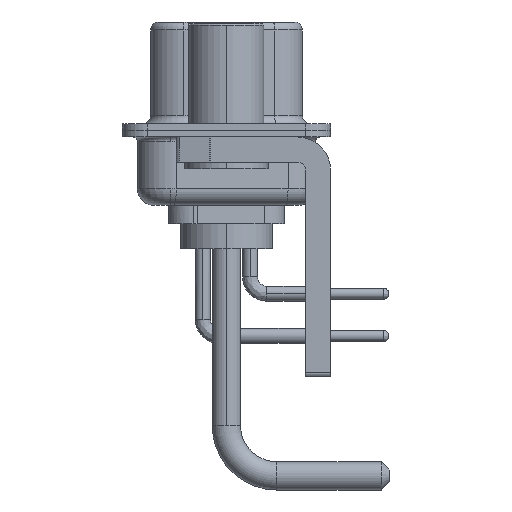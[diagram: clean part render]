
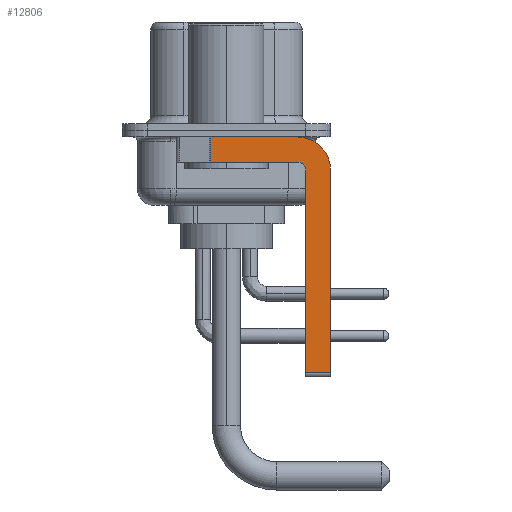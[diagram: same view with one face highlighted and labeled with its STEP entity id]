
A CAD part, left-side view. The second image highlights one B-rep face of the part: STEP entity #12806.
In plain terms, the highlighted planar face has unit normal (-1, 0, 0).
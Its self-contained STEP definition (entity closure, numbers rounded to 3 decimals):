
#111 = VERTEX_POINT ( 'NONE', #14367 ) ;
#200 = VERTEX_POINT ( 'NONE', #21449 ) ;
#1377 = DIRECTION ( 'NONE',  ( 0., -1., 0. ) ) ;
#1684 = CARTESIAN_POINT ( 'NONE',  ( -2.9, -4.75, -14.55 ) ) ;
#1883 = VERTEX_POINT ( 'NONE', #28698 ) ;
#2095 = CARTESIAN_POINT ( 'NONE',  ( -2.9, 0.978, -0.4 ) ) ;
#2115 = AXIS2_PLACEMENT_3D ( 'NONE', #6969, #25020, #13651 ) ;
#2804 = LINE ( 'NONE', #27087, #27906 ) ;
#3168 = ORIENTED_EDGE ( 'NONE', *, *, #22946, .F. ) ;
#3683 = LINE ( 'NONE', #9779, #7607 ) ;
#4151 = VERTEX_POINT ( 'NONE', #1684 ) ;
#4389 = VERTEX_POINT ( 'NONE', #9547 ) ;
#5531 = ORIENTED_EDGE ( 'NONE', *, *, #5847, .F. ) ;
#5847 = EDGE_CURVE ( 'NONE', #4389, #8508, #18278, .T. ) ;
#5997 = CARTESIAN_POINT ( 'NONE',  ( -2.9, 0.978, -1.9 ) ) ;
#6683 = FACE_OUTER_BOUND ( 'NONE', #7619, .T. ) ;
#6900 = CARTESIAN_POINT ( 'NONE',  ( -2.9, -4.25, -1.9 ) ) ;
#6969 = CARTESIAN_POINT ( 'NONE',  ( -2.9, -4.25, -2.4 ) ) ;
#7031 = LINE ( 'NONE', #15608, #28446 ) ;
#7234 = AXIS2_PLACEMENT_3D ( 'NONE', #18364, #13956, #14244 ) ;
#7290 = CARTESIAN_POINT ( 'NONE',  ( -2.9, -6.25, -14.55 ) ) ;
#7607 = VECTOR ( 'NONE', #28403, 1000. ) ;
#7619 = EDGE_LOOP ( 'NONE', ( #13368, #10716, #5531, #3168, #17018, #23373, #12630, #25626 ) ) ;
#8508 = VERTEX_POINT ( 'NONE', #5997 ) ;
#9063 = PLANE ( 'NONE',  #2115 ) ;
#9358 = EDGE_CURVE ( 'NONE', #111, #200, #10565, .T. ) ;
#9547 = CARTESIAN_POINT ( 'NONE',  ( -2.9, -4.25, -1.9 ) ) ;
#9779 = CARTESIAN_POINT ( 'NONE',  ( -2.9, -6.25, -2.4 ) ) ;
#10003 = EDGE_CURVE ( 'NONE', #4151, #19556, #7031, .T. ) ;
#10565 = CIRCLE ( 'NONE', #7234, 2. ) ;
#10716 = ORIENTED_EDGE ( 'NONE', *, *, #17735, .T. ) ;
#11344 = DIRECTION ( 'NONE',  ( 0., -1., 0. ) ) ;
#11863 = DIRECTION ( 'NONE',  ( 0., 0., -1. ) ) ;
#12630 = ORIENTED_EDGE ( 'NONE', *, *, #17860, .F. ) ;
#12806 = ADVANCED_FACE ( 'NONE', ( #6683 ), #9063, .F. ) ;
#13368 = ORIENTED_EDGE ( 'NONE', *, *, #24885, .F. ) ;
#13651 = DIRECTION ( 'NONE',  ( 0., 0., -1. ) ) ;
#13956 = DIRECTION ( 'NONE',  ( 1., 0., 0. ) ) ;
#14244 = DIRECTION ( 'NONE',  ( 0., 0., -1. ) ) ;
#14367 = CARTESIAN_POINT ( 'NONE',  ( -2.9, -4.25, -0.4 ) ) ;
#14396 = LINE ( 'NONE', #26209, #22662 ) ;
#15608 = CARTESIAN_POINT ( 'NONE',  ( -2.9, -4.25, -14.55 ) ) ;
#16412 = VERTEX_POINT ( 'NONE', #2095 ) ;
#17018 = ORIENTED_EDGE ( 'NONE', *, *, #17396, .F. ) ;
#17105 = CARTESIAN_POINT ( 'NONE',  ( -2.9, -4.25, -2.4 ) ) ;
#17396 = EDGE_CURVE ( 'NONE', #4151, #1883, #14396, .T. ) ;
#17735 = EDGE_CURVE ( 'NONE', #16412, #8508, #2804, .T. ) ;
#17860 = EDGE_CURVE ( 'NONE', #200, #19556, #3683, .T. ) ;
#18278 = LINE ( 'NONE', #6900, #19007 ) ;
#18364 = CARTESIAN_POINT ( 'NONE',  ( -2.9, -4.25, -2.4 ) ) ;
#18411 = AXIS2_PLACEMENT_3D ( 'NONE', #17105, #19310, #28213 ) ;
#19007 = VECTOR ( 'NONE', #20198, 1000. ) ;
#19310 = DIRECTION ( 'NONE',  ( -1., 0., 0. ) ) ;
#19423 = LINE ( 'NONE', #26247, #27384 ) ;
#19556 = VERTEX_POINT ( 'NONE', #7290 ) ;
#20198 = DIRECTION ( 'NONE',  ( 0., 1., 0. ) ) ;
#21449 = CARTESIAN_POINT ( 'NONE',  ( -2.9, -6.25, -2.4 ) ) ;
#22194 = CIRCLE ( 'NONE', #18411, 0.5 ) ;
#22662 = VECTOR ( 'NONE', #28006, 1000. ) ;
#22946 = EDGE_CURVE ( 'NONE', #1883, #4389, #22194, .T. ) ;
#23373 = ORIENTED_EDGE ( 'NONE', *, *, #10003, .T. ) ;
#24885 = EDGE_CURVE ( 'NONE', #16412, #111, #19423, .T. ) ;
#25020 = DIRECTION ( 'NONE',  ( 1., 0., 0. ) ) ;
#25626 = ORIENTED_EDGE ( 'NONE', *, *, #9358, .F. ) ;
#26209 = CARTESIAN_POINT ( 'NONE',  ( -2.9, -4.75, -14.8 ) ) ;
#26247 = CARTESIAN_POINT ( 'NONE',  ( -2.9, 3., -0.4 ) ) ;
#27087 = CARTESIAN_POINT ( 'NONE',  ( -2.9, 0.978, -1.9 ) ) ;
#27384 = VECTOR ( 'NONE', #1377, 1000. ) ;
#27906 = VECTOR ( 'NONE', #11863, 1000. ) ;
#28006 = DIRECTION ( 'NONE',  ( 0., 0., 1. ) ) ;
#28213 = DIRECTION ( 'NONE',  ( 0., 0., 1. ) ) ;
#28403 = DIRECTION ( 'NONE',  ( 0., 0., -1. ) ) ;
#28446 = VECTOR ( 'NONE', #11344, 1000. ) ;
#28698 = CARTESIAN_POINT ( 'NONE',  ( -2.9, -4.75, -2.4 ) ) ;
